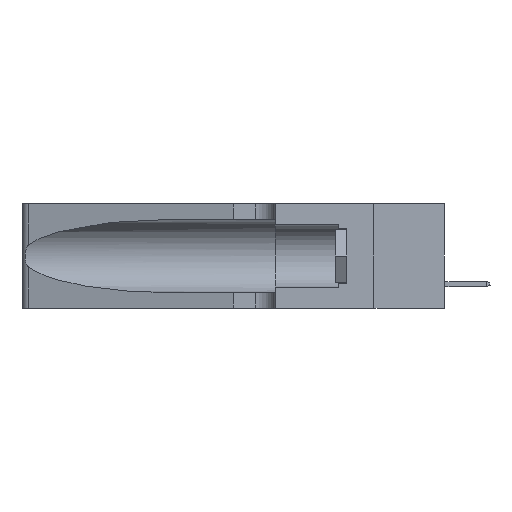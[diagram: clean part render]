
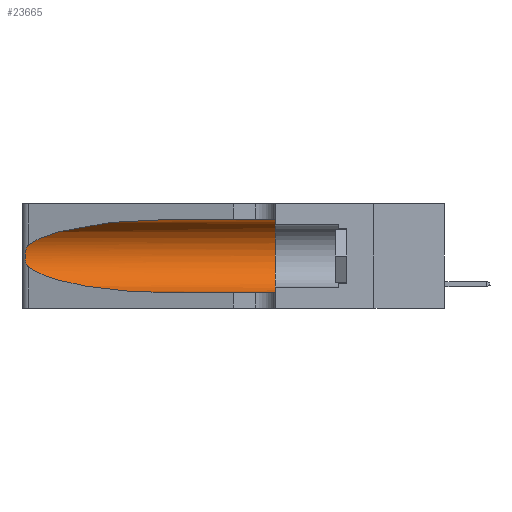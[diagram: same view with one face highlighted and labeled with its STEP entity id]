
A CAD part, left-side view. The second image highlights one B-rep face of the part: STEP entity #23665.
In plain terms, the highlighted cylindrical face has radius 3.308 mm (diameter 6.617 mm), a partial arc.
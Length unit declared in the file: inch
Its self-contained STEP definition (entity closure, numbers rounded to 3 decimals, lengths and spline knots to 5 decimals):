
#354 = CARTESIAN_POINT ( 'NONE',  ( 0.25487, 1.22718, 0.14631 ) ) ;
#1000 = CARTESIAN_POINT ( 'NONE',  ( 0.1305, 1.61858, 0.31525 ) ) ;
#1518 = EDGE_CURVE ( 'NONE', #6913, #8010, #7608, .T. ) ;
#1672 = EDGE_CURVE ( 'NONE', #8171, #6913, #17846, .T. ) ;
#1764 = AXIS2_PLACEMENT_3D ( 'NONE', #16467, #3379, #18634 ) ;
#2940 = B_SPLINE_CURVE_WITH_KNOTS ( 'NONE', 3,
 ( #21844, #15093, #10878, #28057, #26137, #19809, #14996, #4133, #19365, #6311, #21566, #8512, #17946, #354 ),
 .UNSPECIFIED., .F., .F.,
 ( 4, 2, 2, 2, 2, 2, 4 ),
 ( 0., 0.00027, 0.00053, 0.00107, 0.0016, 0.00187, 0.00214 ),
 .UNSPECIFIED. ) ;
#3081 = VERTEX_POINT ( 'NONE', #10812 ) ;
#3379 = DIRECTION ( 'NONE',  ( 0., -1., 0. ) ) ;
#3841 = ORIENTED_EDGE ( 'NONE', *, *, #25538, .T. ) ;
#4133 = CARTESIAN_POINT ( 'NONE',  ( 0.26075, 1.23896, 0.178 ) ) ;
#4180 = LINE ( 'NONE', #16282, #8602 ) ;
#4898 = AXIS2_PLACEMENT_3D ( 'NONE', #9152, #11437, #11537 ) ;
#6311 = CARTESIAN_POINT ( 'NONE',  ( 0.25856, 1.23593, 0.16098 ) ) ;
#6326 = EDGE_CURVE ( 'NONE', #20039, #19524, #20392, .T. ) ;
#6913 = VERTEX_POINT ( 'NONE', #26632 ) ;
#7295 = CARTESIAN_POINT ( 'NONE',  ( 0.18966, 0.96281, 0.31525 ) ) ;
#7608 = CIRCLE ( 'NONE', #4898, 0.13025 ) ;
#7727 = CARTESIAN_POINT ( 'NONE',  ( 0.25487, 1.22718, 0.14631 ) ) ;
#8010 = VERTEX_POINT ( 'NONE', #17598 ) ;
#8171 = VERTEX_POINT ( 'NONE', #20506 ) ;
#8512 = CARTESIAN_POINT ( 'NONE',  ( 0.25639, 1.23186, 0.15144 ) ) ;
#8602 = VECTOR ( 'NONE', #13869, 39.37008 ) ;
#8670 = EDGE_CURVE ( 'NONE', #19524, #8010, #4180, .T. ) ;
#9152 = CARTESIAN_POINT ( 'NONE',  ( 0.1305, 0.35, 0.185 ) ) ;
#9822 = CARTESIAN_POINT ( 'NONE',  ( 0.25487, 1.22718, 0.14631 ) ) ;
#9999 = ORIENTED_EDGE ( 'NONE', *, *, #26819, .T. ) ;
#10812 = CARTESIAN_POINT ( 'NONE',  ( 0.25487, 1.22718, 0.22369 ) ) ;
#10878 = CARTESIAN_POINT ( 'NONE',  ( 0.25639, 1.23184, 0.21858 ) ) ;
#11194 = CARTESIAN_POINT ( 'NONE',  ( 0.2373, 1.15595, 0.28018 ) ) ;
#11437 = DIRECTION ( 'NONE',  ( 0., 1., 0. ) ) ;
#11537 = DIRECTION ( 'NONE',  ( 0., 0., 1. ) ) ;
#13869 = DIRECTION ( 'NONE',  ( 0., -1., 0. ) ) ;
#14821 = CYLINDRICAL_SURFACE ( 'NONE', #1764, 0.13025 ) ;
#14996 = CARTESIAN_POINT ( 'NONE',  ( 0.26075, 1.23896, 0.19203 ) ) ;
#15093 = CARTESIAN_POINT ( 'NONE',  ( 0.25555, 1.22994, 0.2215 ) ) ;
#16282 = CARTESIAN_POINT ( 'NONE',  ( 0.1305, 1.61858, 0.05475 ) ) ;
#16467 = CARTESIAN_POINT ( 'NONE',  ( 0.1305, 1.61858, 0.185 ) ) ;
#16493 = ORIENTED_EDGE ( 'NONE', *, *, #8670, .T. ) ;
#16514 = EDGE_LOOP ( 'NONE', ( #9999, #3841, #26610, #16493, #18241, #22824 ) ) ;
#17598 = CARTESIAN_POINT ( 'NONE',  ( 0.1305, 0.35, 0.05475 ) ) ;
#17846 = LINE ( 'NONE', #1000, #21578 ) ;
#17946 = CARTESIAN_POINT ( 'NONE',  ( 0.25555, 1.22993, 0.14849 ) ) ;
#18241 = ORIENTED_EDGE ( 'NONE', *, *, #1518, .F. ) ;
#18634 = DIRECTION ( 'NONE',  ( 0., 0., -1. ) ) ;
#18671 = CARTESIAN_POINT ( 'NONE',  ( 0.2373, 1.15595, 0.08982 ) ) ;
#19365 = CARTESIAN_POINT ( 'NONE',  ( 0.26017, 1.23833, 0.17102 ) ) ;
#19524 = VERTEX_POINT ( 'NONE', #27535 ) ;
#19676 = CARTESIAN_POINT ( 'NONE',  ( 0.25487, 1.22718, 0.22369 ) ) ;
#19809 = CARTESIAN_POINT ( 'NONE',  ( 0.26018, 1.23835, 0.19895 ) ) ;
#20039 = VERTEX_POINT ( 'NONE', #7727 ) ;
#20392 =( BOUNDED_CURVE ( )  B_SPLINE_CURVE ( 3, ( #9822, #18671, #28185, #25010 ),
 .UNSPECIFIED., .F., .T. ) 
 B_SPLINE_CURVE_WITH_KNOTS ( ( 4, 4 ),
 ( 3.44316, 4.71239 ),
 .UNSPECIFIED. ) 
 CURVE ( )  GEOMETRIC_REPRESENTATION_ITEM ( )  RATIONAL_B_SPLINE_CURVE ( ( 1., 0.87, 0.87, 1. ) ) 
 REPRESENTATION_ITEM ( '' )  );
#20506 = CARTESIAN_POINT ( 'NONE',  ( 0.1305, 0.72297, 0.31525 ) ) ;
#21566 = CARTESIAN_POINT ( 'NONE',  ( 0.25789, 1.23486, 0.15765 ) ) ;
#21578 = VECTOR ( 'NONE', #27142, 39.37008 ) ;
#21844 = CARTESIAN_POINT ( 'NONE',  ( 0.25487, 1.22718, 0.22369 ) ) ;
#22824 = ORIENTED_EDGE ( 'NONE', *, *, #1672, .F. ) ;
#23012 = FACE_OUTER_BOUND ( 'NONE', #16514, .T. ) ;
#23665 = ADVANCED_FACE ( 'NONE', ( #23012 ), #14821, .F. ) ;
#24063 = CARTESIAN_POINT ( 'NONE',  ( 0.1305, 0.72297, 0.31525 ) ) ;
#25010 = CARTESIAN_POINT ( 'NONE',  ( 0.1305, 0.72297, 0.05475 ) ) ;
#25538 = EDGE_CURVE ( 'NONE', #3081, #20039, #2940, .T. ) ;
#26137 = CARTESIAN_POINT ( 'NONE',  ( 0.25854, 1.2359, 0.20912 ) ) ;
#26610 = ORIENTED_EDGE ( 'NONE', *, *, #6326, .T. ) ;
#26632 = CARTESIAN_POINT ( 'NONE',  ( 0.1305, 0.35, 0.31525 ) ) ;
#26689 =( BOUNDED_CURVE ( )  B_SPLINE_CURVE ( 3, ( #24063, #7295, #11194, #19676 ),
 .UNSPECIFIED., .F., .F. ) 
 B_SPLINE_CURVE_WITH_KNOTS ( ( 4, 4 ),
 ( 1.5708, 2.84003 ),
 .UNSPECIFIED. ) 
 CURVE ( )  GEOMETRIC_REPRESENTATION_ITEM ( )  RATIONAL_B_SPLINE_CURVE ( ( 1., 0.87, 0.87, 1. ) ) 
 REPRESENTATION_ITEM ( '' )  );
#26819 = EDGE_CURVE ( 'NONE', #8171, #3081, #26689, .T. ) ;
#27142 = DIRECTION ( 'NONE',  ( 0., -1., 0. ) ) ;
#27535 = CARTESIAN_POINT ( 'NONE',  ( 0.1305, 0.72297, 0.05475 ) ) ;
#28057 = CARTESIAN_POINT ( 'NONE',  ( 0.25787, 1.23484, 0.2124 ) ) ;
#28185 = CARTESIAN_POINT ( 'NONE',  ( 0.18966, 0.96281, 0.05475 ) ) ;
